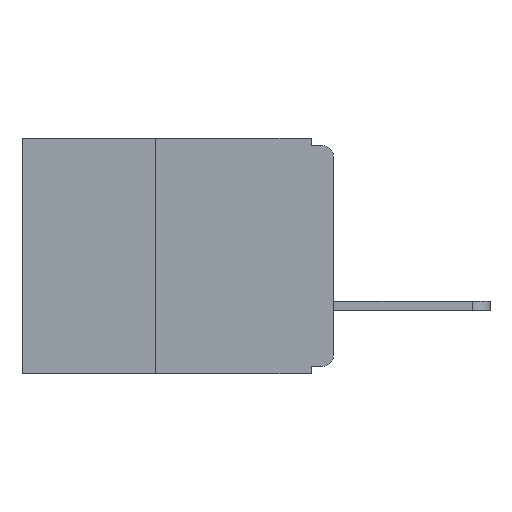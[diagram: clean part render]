
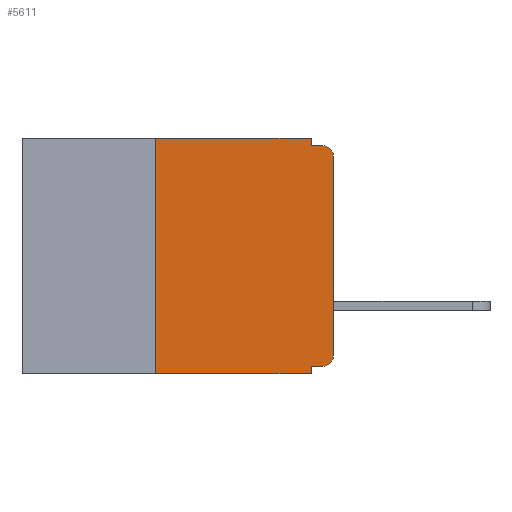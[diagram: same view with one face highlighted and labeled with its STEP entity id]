
A CAD part, left-side view. The second image highlights one B-rep face of the part: STEP entity #5611.
In plain terms, the highlighted planar face has unit normal (-1, 0, 0).
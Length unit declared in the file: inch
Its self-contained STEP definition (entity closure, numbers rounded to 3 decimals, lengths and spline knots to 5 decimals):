
#96 = DIRECTION ( 'NONE',  ( 0., 1., 0. ) ) ;
#164 = CARTESIAN_POINT ( 'NONE',  ( 0., 0., -0.32 ) ) ;
#265 = LINE ( 'NONE', #18371, #25496 ) ;
#286 = EDGE_CURVE ( 'NONE', #11356, #13684, #25078, .T. ) ;
#850 = CARTESIAN_POINT ( 'NONE',  ( 0., 0.015, -0.025 ) ) ;
#961 = DIRECTION ( 'NONE',  ( 0., 0., 1. ) ) ;
#1650 = EDGE_LOOP ( 'NONE', ( #19714, #24700, #24995, #18850, #13398, #6785, #19553, #9028, #27203, #7361 ) ) ;
#2409 = FACE_OUTER_BOUND ( 'NONE', #1650, .T. ) ;
#2808 = CARTESIAN_POINT ( 'NONE',  ( 0., 0., -0.01 ) ) ;
#2827 = PLANE ( 'NONE',  #12642 ) ;
#3039 = VERTEX_POINT ( 'NONE', #16902 ) ;
#3173 = DIRECTION ( 'NONE',  ( 0., 0., -1. ) ) ;
#3200 = VERTEX_POINT ( 'NONE', #12960 ) ;
#4024 = CIRCLE ( 'NONE', #28135, 0.015 ) ;
#4375 = EDGE_CURVE ( 'NONE', #3200, #15040, #14782, .T. ) ;
#4548 = DIRECTION ( 'NONE',  ( 0., -1., 0. ) ) ;
#4648 = DIRECTION ( 'NONE',  ( 0., 0., 1. ) ) ;
#4780 = CARTESIAN_POINT ( 'NONE',  ( 0., 0., -0.025 ) ) ;
#4953 = CARTESIAN_POINT ( 'NONE',  ( 0., 0.25, 0. ) ) ;
#5196 = EDGE_CURVE ( 'NONE', #13684, #3039, #26941, .T. ) ;
#5566 = VECTOR ( 'NONE', #18830, 39.37008 ) ;
#5611 = ADVANCED_FACE ( 'NONE', ( #2409 ), #2827, .F. ) ;
#6785 = ORIENTED_EDGE ( 'NONE', *, *, #25023, .F. ) ;
#7361 = ORIENTED_EDGE ( 'NONE', *, *, #10117, .T. ) ;
#7433 = CARTESIAN_POINT ( 'NONE',  ( 0., 0.437, 0. ) ) ;
#8030 = VECTOR ( 'NONE', #21656, 39.37008 ) ;
#8782 = CIRCLE ( 'NONE', #14840, 0.015 ) ;
#8828 = CARTESIAN_POINT ( 'NONE',  ( 0., 0.031, -0.01 ) ) ;
#9028 = ORIENTED_EDGE ( 'NONE', *, *, #5196, .F. ) ;
#9397 = EDGE_CURVE ( 'NONE', #20360, #28030, #11742, .T. ) ;
#9940 = VECTOR ( 'NONE', #4648, 39.37008 ) ;
#10117 = EDGE_CURVE ( 'NONE', #11356, #3200, #8782, .T. ) ;
#10582 = CARTESIAN_POINT ( 'NONE',  ( 0., 0.031, -0.32 ) ) ;
#11356 = VERTEX_POINT ( 'NONE', #18698 ) ;
#11742 = LINE ( 'NONE', #11785, #5566 ) ;
#11785 = CARTESIAN_POINT ( 'NONE',  ( 0., 0.437, 0. ) ) ;
#12326 = CARTESIAN_POINT ( 'NONE',  ( 0., 0.015, -0.305 ) ) ;
#12642 = AXIS2_PLACEMENT_3D ( 'NONE', #7433, #28145, #14436 ) ;
#12795 = LINE ( 'NONE', #19355, #8030 ) ;
#12853 = VECTOR ( 'NONE', #96, 39.37008 ) ;
#12960 = CARTESIAN_POINT ( 'NONE',  ( 0., 0., -0.305 ) ) ;
#13398 = ORIENTED_EDGE ( 'NONE', *, *, #9397, .F. ) ;
#13684 = VERTEX_POINT ( 'NONE', #10582 ) ;
#13875 = EDGE_CURVE ( 'NONE', #27664, #3039, #265, .T. ) ;
#14436 = DIRECTION ( 'NONE',  ( 0., 0., -1. ) ) ;
#14644 = DIRECTION ( 'NONE',  ( 0., 0., -1. ) ) ;
#14782 = LINE ( 'NONE', #28505, #26254 ) ;
#14840 = AXIS2_PLACEMENT_3D ( 'NONE', #12326, #28357, #14644 ) ;
#15040 = VERTEX_POINT ( 'NONE', #4780 ) ;
#15783 = EDGE_CURVE ( 'NONE', #18811, #23733, #16420, .T. ) ;
#16420 = LINE ( 'NONE', #2808, #27855 ) ;
#16663 = DIRECTION ( 'NONE',  ( 0., -1., 0. ) ) ;
#16902 = CARTESIAN_POINT ( 'NONE',  ( 0., 0.031, -0.33 ) ) ;
#16975 = CARTESIAN_POINT ( 'NONE',  ( 0., 0.25, -0.33 ) ) ;
#16997 = DIRECTION ( 'NONE',  ( -1., 0., 0. ) ) ;
#17900 = EDGE_CURVE ( 'NONE', #15040, #23733, #4024, .T. ) ;
#18371 = CARTESIAN_POINT ( 'NONE',  ( 0., 0.437, -0.33 ) ) ;
#18698 = CARTESIAN_POINT ( 'NONE',  ( 0., 0.015, -0.32 ) ) ;
#18811 = VERTEX_POINT ( 'NONE', #8828 ) ;
#18830 = DIRECTION ( 'NONE',  ( 0., -1., 0. ) ) ;
#18850 = ORIENTED_EDGE ( 'NONE', *, *, #27059, .F. ) ;
#19355 = CARTESIAN_POINT ( 'NONE',  ( 0., 0.031, 0. ) ) ;
#19553 = ORIENTED_EDGE ( 'NONE', *, *, #13875, .T. ) ;
#19714 = ORIENTED_EDGE ( 'NONE', *, *, #4375, .T. ) ;
#19895 = DIRECTION ( 'NONE',  ( 0., 0., -1. ) ) ;
#20360 = VERTEX_POINT ( 'NONE', #4953 ) ;
#20583 = CARTESIAN_POINT ( 'NONE',  ( 0., 0.015, -0.01 ) ) ;
#21656 = DIRECTION ( 'NONE',  ( 0., 0., -1. ) ) ;
#23105 = CARTESIAN_POINT ( 'NONE',  ( 0., 0.25, -0.33 ) ) ;
#23733 = VERTEX_POINT ( 'NONE', #20583 ) ;
#24423 = CARTESIAN_POINT ( 'NONE',  ( 0., 0.031, -0.33 ) ) ;
#24700 = ORIENTED_EDGE ( 'NONE', *, *, #17900, .T. ) ;
#24995 = ORIENTED_EDGE ( 'NONE', *, *, #15783, .F. ) ;
#25023 = EDGE_CURVE ( 'NONE', #27664, #20360, #28275, .T. ) ;
#25078 = LINE ( 'NONE', #164, #12853 ) ;
#25496 = VECTOR ( 'NONE', #4548, 39.37008 ) ;
#25498 = VECTOR ( 'NONE', #19895, 39.37008 ) ;
#26254 = VECTOR ( 'NONE', #961, 39.37008 ) ;
#26941 = LINE ( 'NONE', #24423, #25498 ) ;
#27059 = EDGE_CURVE ( 'NONE', #28030, #18811, #12795, .T. ) ;
#27203 = ORIENTED_EDGE ( 'NONE', *, *, #286, .F. ) ;
#27664 = VERTEX_POINT ( 'NONE', #16975 ) ;
#27855 = VECTOR ( 'NONE', #16663, 39.37008 ) ;
#28030 = VERTEX_POINT ( 'NONE', #29717 ) ;
#28135 = AXIS2_PLACEMENT_3D ( 'NONE', #850, #16997, #3173 ) ;
#28145 = DIRECTION ( 'NONE',  ( 1., 0., 0. ) ) ;
#28275 = LINE ( 'NONE', #23105, #9940 ) ;
#28357 = DIRECTION ( 'NONE',  ( -1., 0., 0. ) ) ;
#28505 = CARTESIAN_POINT ( 'NONE',  ( 0., 0., 0. ) ) ;
#29717 = CARTESIAN_POINT ( 'NONE',  ( 0., 0.031, 0. ) ) ;
